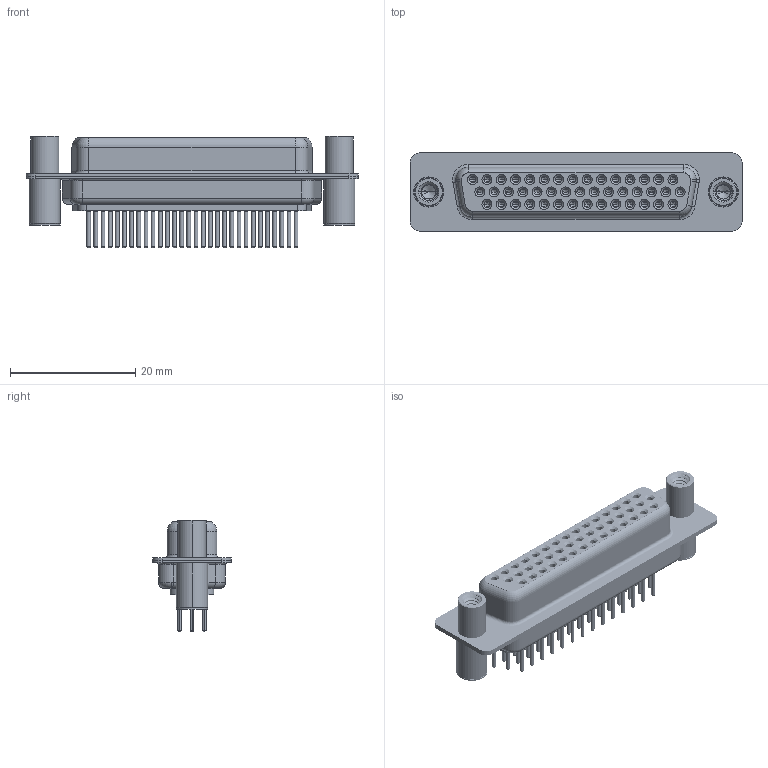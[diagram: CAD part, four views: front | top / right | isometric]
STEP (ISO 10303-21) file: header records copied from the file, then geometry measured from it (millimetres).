
FILE_DESCRIPTION (( 'STEP AP203' ), '1' );
FILE_NAME ('638-M44-630-BT4.STEP', '2022-07-05T20:51:32', ( '' ), ( '' ), 'SwSTEP 2.0', 'SolidWorks 2020', '' );
FILE_SCHEMA (( 'CONFIG_CONTROL_DESIGN' ));
Length unit declared in the file: millimetre
Products named in the file (8): 638M Contact Row 1_30; 638M Shell Front_44 Contacts; 638M Contact Row 2_30; 638-M44-630-BT4; 638M Housing_44 Contacts; 638M Contact Row 3_30; 638M 4-40 Threaded Standoff and Board Spacer; 638M Shell Rear_44 Contacts
Assembly tree (49 placements, depth 2):
  638-M44-630-BT4
    638M Housing_44 Contacts
    638M Shell Front_44 Contacts
    638M Shell Rear_44 Contacts
    638M Contact Row 1_30  x15
    638M Contact Row 2_30  x15
    638M Contact Row 3_30  x14
    638M 4-40 Threaded Standoff and Board Spacer  x2
Bounding box: 53.05 x 12.5 x 17.8 mm (x, y, z)
Volume: 3822.9 mm3; surface area: 12548.2 mm2
Topology: 49 solids, 49 shells, 2785 faces, 6455 edges, 3953 vertices
Faces by surface type: cylinder 1025, plane 733, torus 677, cone 338, bspline 12
Entity records: 32444 total; most frequent: CARTESIAN_POINT 7176, DIRECTION 5414, ORIENTED_EDGE 4466, AXIS2_PLACEMENT_3D 2302, EDGE_CURVE 2233, VERTEX_POINT 1413, CIRCLE 1269, EDGE_LOOP 1240
